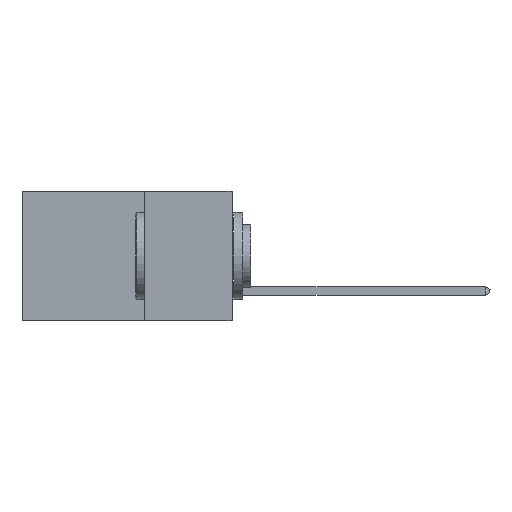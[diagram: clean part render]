
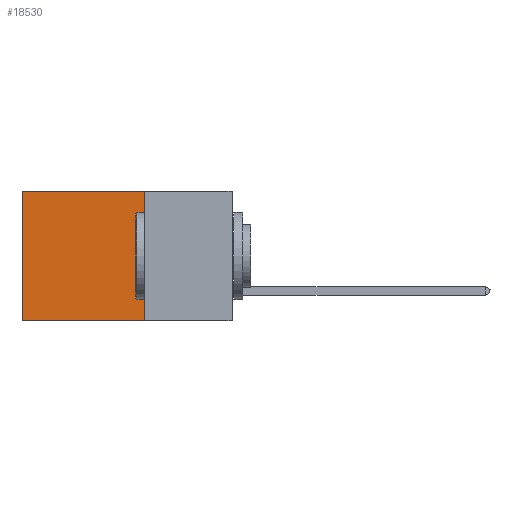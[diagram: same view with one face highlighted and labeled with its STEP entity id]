
A CAD part, left-side view. The second image highlights one B-rep face of the part: STEP entity #18530.
In plain terms, the highlighted planar face has unit normal (-1, 0, 0).
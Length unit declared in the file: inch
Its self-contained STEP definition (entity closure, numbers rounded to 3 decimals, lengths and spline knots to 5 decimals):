
#898 = VECTOR ( 'NONE', #31617, 39.37008 ) ;
#1921 = VECTOR ( 'NONE', #17488, 39.37008 ) ;
#2423 = CARTESIAN_POINT ( 'NONE',  ( 0.2875, 0.6, 0. ) ) ;
#2572 = DIRECTION ( 'NONE',  ( 1., 0., 0. ) ) ;
#2582 = CARTESIAN_POINT ( 'NONE',  ( 0.2875, 0.25, 0. ) ) ;
#3770 = VERTEX_POINT ( 'NONE', #30682 ) ;
#6088 = ORIENTED_EDGE ( 'NONE', *, *, #11930, .F. ) ;
#8272 = ORIENTED_EDGE ( 'NONE', *, *, #10181, .T. ) ;
#10181 = EDGE_CURVE ( 'NONE', #12716, #3770, #15471, .T. ) ;
#11930 = EDGE_CURVE ( 'NONE', #22906, #23765, #18463, .T. ) ;
#12716 = VERTEX_POINT ( 'NONE', #27628 ) ;
#15471 = LINE ( 'NONE', #2423, #898 ) ;
#16048 = DIRECTION ( 'NONE',  ( 0., 0., -1. ) ) ;
#16219 = FACE_OUTER_BOUND ( 'NONE', #29780, .T. ) ;
#16441 = ORIENTED_EDGE ( 'NONE', *, *, #20099, .F. ) ;
#17488 = DIRECTION ( 'NONE',  ( 0., 1., 0. ) ) ;
#18463 = LINE ( 'NONE', #19386, #29164 ) ;
#18530 = ADVANCED_FACE ( 'NONE', ( #16219 ), #30749, .F. ) ;
#18794 = ORIENTED_EDGE ( 'NONE', *, *, #20333, .T. ) ;
#19056 = DIRECTION ( 'NONE',  ( 0., 0., -1. ) ) ;
#19386 = CARTESIAN_POINT ( 'NONE',  ( 0.2875, 0.25, 0. ) ) ;
#20099 = EDGE_CURVE ( 'NONE', #23765, #3770, #20739, .T. ) ;
#20333 = EDGE_CURVE ( 'NONE', #22906, #12716, #20707, .T. ) ;
#20707 = LINE ( 'NONE', #2582, #1921 ) ;
#20739 = LINE ( 'NONE', #29567, #24887 ) ;
#21997 = DIRECTION ( 'NONE',  ( 0., 1., 0. ) ) ;
#22906 = VERTEX_POINT ( 'NONE', #28683 ) ;
#23765 = VERTEX_POINT ( 'NONE', #23905 ) ;
#23905 = CARTESIAN_POINT ( 'NONE',  ( 0.2875, 0.25, -0.37 ) ) ;
#24887 = VECTOR ( 'NONE', #21997, 39.37008 ) ;
#26599 = AXIS2_PLACEMENT_3D ( 'NONE', #30852, #2572, #16048 ) ;
#27628 = CARTESIAN_POINT ( 'NONE',  ( 0.2875, 0.6, 0. ) ) ;
#28683 = CARTESIAN_POINT ( 'NONE',  ( 0.2875, 0.25, 0. ) ) ;
#29164 = VECTOR ( 'NONE', #19056, 39.37008 ) ;
#29567 = CARTESIAN_POINT ( 'NONE',  ( 0.2875, 0.25, -0.37 ) ) ;
#29780 = EDGE_LOOP ( 'NONE', ( #8272, #16441, #6088, #18794 ) ) ;
#30682 = CARTESIAN_POINT ( 'NONE',  ( 0.2875, 0.6, -0.37 ) ) ;
#30749 = PLANE ( 'NONE',  #26599 ) ;
#30852 = CARTESIAN_POINT ( 'NONE',  ( 0.2875, 0.25, 0. ) ) ;
#31617 = DIRECTION ( 'NONE',  ( 0., 0., -1. ) ) ;
